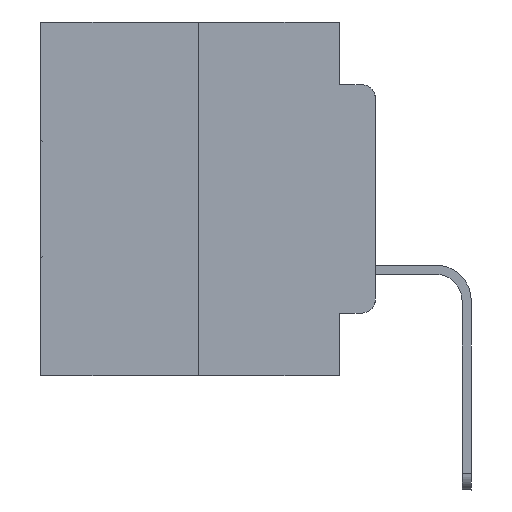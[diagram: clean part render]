
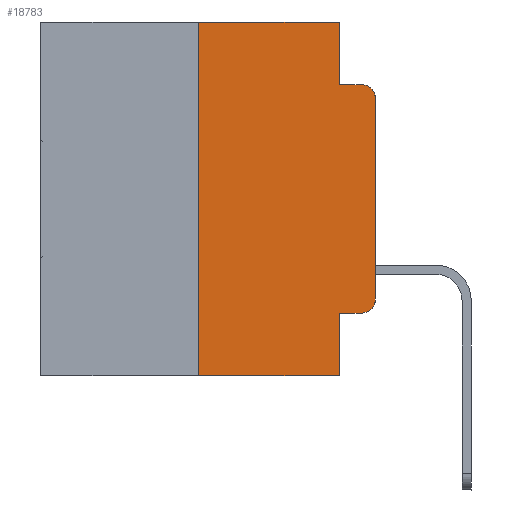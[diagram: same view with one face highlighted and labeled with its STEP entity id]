
A CAD part, left-side view. The second image highlights one B-rep face of the part: STEP entity #18783.
In plain terms, the highlighted planar face has unit normal (-1, 0, 0).
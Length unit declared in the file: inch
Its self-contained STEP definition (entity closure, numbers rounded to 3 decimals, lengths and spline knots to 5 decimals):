
#6 = CARTESIAN_POINT ( 'NONE',  ( 0., 0.051, -0.0885 ) ) ;
#219 = CARTESIAN_POINT ( 'NONE',  ( 0., 0., 0. ) ) ;
#548 = AXIS2_PLACEMENT_3D ( 'NONE', #17160, #19523, #12802 ) ;
#899 = DIRECTION ( 'NONE',  ( 0., -1., 0. ) ) ;
#1020 = DIRECTION ( 'NONE',  ( -1., 0., 0. ) ) ;
#1212 = CARTESIAN_POINT ( 'NONE',  ( 0., 0.051, -0.4115 ) ) ;
#1328 = VERTEX_POINT ( 'NONE', #11670 ) ;
#1495 = CARTESIAN_POINT ( 'NONE',  ( 0., 0.051, 0. ) ) ;
#1775 = CARTESIAN_POINT ( 'NONE',  ( 0., 0.25, 0. ) ) ;
#1780 = ORIENTED_EDGE ( 'NONE', *, *, #18916, .T. ) ;
#2362 = LINE ( 'NONE', #15969, #4985 ) ;
#3012 = DIRECTION ( 'NONE',  ( 0., 0., -1. ) ) ;
#3477 = DIRECTION ( 'NONE',  ( 0., -1., 0. ) ) ;
#3526 = DIRECTION ( 'NONE',  ( 0., -1., 0. ) ) ;
#3650 = EDGE_CURVE ( 'NONE', #14649, #15134, #19841, .T. ) ;
#4070 = LINE ( 'NONE', #219, #11869 ) ;
#4186 = DIRECTION ( 'NONE',  ( 0., 0., -1. ) ) ;
#4557 = ORIENTED_EDGE ( 'NONE', *, *, #26781, .F. ) ;
#4600 = VECTOR ( 'NONE', #899, 39.37008 ) ;
#4755 = ORIENTED_EDGE ( 'NONE', *, *, #3650, .T. ) ;
#4985 = VECTOR ( 'NONE', #20918, 39.37008 ) ;
#5054 = VERTEX_POINT ( 'NONE', #6 ) ;
#5147 = VECTOR ( 'NONE', #7427, 39.37008 ) ;
#5282 = DIRECTION ( 'NONE',  ( 1., 0., 0. ) ) ;
#5493 = PLANE ( 'NONE',  #11148 ) ;
#5795 = FACE_OUTER_BOUND ( 'NONE', #25592, .T. ) ;
#6465 = VERTEX_POINT ( 'NONE', #18492 ) ;
#7427 = DIRECTION ( 'NONE',  ( 0., -1., 0. ) ) ;
#7872 = CARTESIAN_POINT ( 'NONE',  ( 0., 0.051, 0. ) ) ;
#8125 = EDGE_CURVE ( 'NONE', #17326, #14649, #22370, .T. ) ;
#8355 = CARTESIAN_POINT ( 'NONE',  ( 0., 0.051, -0.0885 ) ) ;
#8402 = CARTESIAN_POINT ( 'NONE',  ( 0., 0., -0.3915 ) ) ;
#9390 = CARTESIAN_POINT ( 'NONE',  ( 0., 0.473, 0. ) ) ;
#9501 = VERTEX_POINT ( 'NONE', #1775 ) ;
#9854 = VECTOR ( 'NONE', #3526, 39.37008 ) ;
#9980 = LINE ( 'NONE', #9390, #5147 ) ;
#10697 = CARTESIAN_POINT ( 'NONE',  ( 0., 0.473, -0.5 ) ) ;
#11148 = AXIS2_PLACEMENT_3D ( 'NONE', #17198, #5282, #3012 ) ;
#11670 = CARTESIAN_POINT ( 'NONE',  ( 0., 0.02, -0.0885 ) ) ;
#11741 = EDGE_CURVE ( 'NONE', #16028, #9501, #2362, .T. ) ;
#11869 = VECTOR ( 'NONE', #28688, 39.37008 ) ;
#12210 = VERTEX_POINT ( 'NONE', #7872 ) ;
#12293 = ORIENTED_EDGE ( 'NONE', *, *, #28412, .F. ) ;
#12802 = DIRECTION ( 'NONE',  ( 0., 0., -1. ) ) ;
#13805 = DIRECTION ( 'NONE',  ( 0., 0., -1. ) ) ;
#14543 = LINE ( 'NONE', #1495, #25994 ) ;
#14649 = VERTEX_POINT ( 'NONE', #27970 ) ;
#14734 = EDGE_CURVE ( 'NONE', #12210, #5054, #24469, .T. ) ;
#14828 = EDGE_CURVE ( 'NONE', #15134, #6465, #4070, .T. ) ;
#14941 = ORIENTED_EDGE ( 'NONE', *, *, #14828, .T. ) ;
#15016 = AXIS2_PLACEMENT_3D ( 'NONE', #15314, #1020, #17591 ) ;
#15134 = VERTEX_POINT ( 'NONE', #8402 ) ;
#15314 = CARTESIAN_POINT ( 'NONE',  ( 0., 0.02, -0.3915 ) ) ;
#15718 = EDGE_CURVE ( 'NONE', #6465, #1328, #17367, .T. ) ;
#15969 = CARTESIAN_POINT ( 'NONE',  ( 0., 0.25, 0. ) ) ;
#16028 = VERTEX_POINT ( 'NONE', #27997 ) ;
#17160 = CARTESIAN_POINT ( 'NONE',  ( 0., 0.02, -0.1085 ) ) ;
#17198 = CARTESIAN_POINT ( 'NONE',  ( 0., 0.473, 0. ) ) ;
#17326 = VERTEX_POINT ( 'NONE', #24457 ) ;
#17367 = CIRCLE ( 'NONE', #548, 0.02 ) ;
#17591 = DIRECTION ( 'NONE',  ( 0., 0., -1. ) ) ;
#17821 = ORIENTED_EDGE ( 'NONE', *, *, #11741, .F. ) ;
#17870 = ORIENTED_EDGE ( 'NONE', *, *, #15718, .T. ) ;
#18492 = CARTESIAN_POINT ( 'NONE',  ( 0., 0., -0.1085 ) ) ;
#18691 = ORIENTED_EDGE ( 'NONE', *, *, #8125, .T. ) ;
#18783 = ADVANCED_FACE ( 'NONE', ( #5795 ), #5493, .F. ) ;
#18916 = EDGE_CURVE ( 'NONE', #16028, #28800, #19832, .T. ) ;
#19523 = DIRECTION ( 'NONE',  ( -1., 0., 0. ) ) ;
#19832 = LINE ( 'NONE', #10697, #9854 ) ;
#19841 = CIRCLE ( 'NONE', #15016, 0.02 ) ;
#20079 = LINE ( 'NONE', #8355, #24900 ) ;
#20918 = DIRECTION ( 'NONE',  ( 0., 0., 1. ) ) ;
#22370 = LINE ( 'NONE', #1212, #4600 ) ;
#22540 = ORIENTED_EDGE ( 'NONE', *, *, #26964, .F. ) ;
#23354 = VECTOR ( 'NONE', #13805, 39.37008 ) ;
#24369 = ORIENTED_EDGE ( 'NONE', *, *, #14734, .F. ) ;
#24457 = CARTESIAN_POINT ( 'NONE',  ( 0., 0.051, -0.4115 ) ) ;
#24469 = LINE ( 'NONE', #25391, #23354 ) ;
#24900 = VECTOR ( 'NONE', #3477, 39.37008 ) ;
#25391 = CARTESIAN_POINT ( 'NONE',  ( 0., 0.051, 0. ) ) ;
#25592 = EDGE_LOOP ( 'NONE', ( #14941, #17870, #4557, #24369, #12293, #17821, #1780, #22540, #18691, #4755 ) ) ;
#25994 = VECTOR ( 'NONE', #4186, 39.37008 ) ;
#26781 = EDGE_CURVE ( 'NONE', #5054, #1328, #20079, .T. ) ;
#26964 = EDGE_CURVE ( 'NONE', #17326, #28800, #14543, .T. ) ;
#27970 = CARTESIAN_POINT ( 'NONE',  ( 0., 0.02, -0.4115 ) ) ;
#27997 = CARTESIAN_POINT ( 'NONE',  ( 0., 0.25, -0.5 ) ) ;
#28412 = EDGE_CURVE ( 'NONE', #9501, #12210, #9980, .T. ) ;
#28688 = DIRECTION ( 'NONE',  ( 0., 0., 1. ) ) ;
#28800 = VERTEX_POINT ( 'NONE', #29966 ) ;
#29966 = CARTESIAN_POINT ( 'NONE',  ( 0., 0.051, -0.5 ) ) ;
